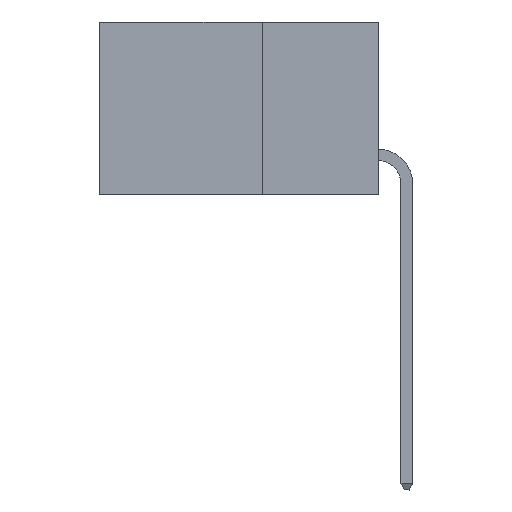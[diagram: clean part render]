
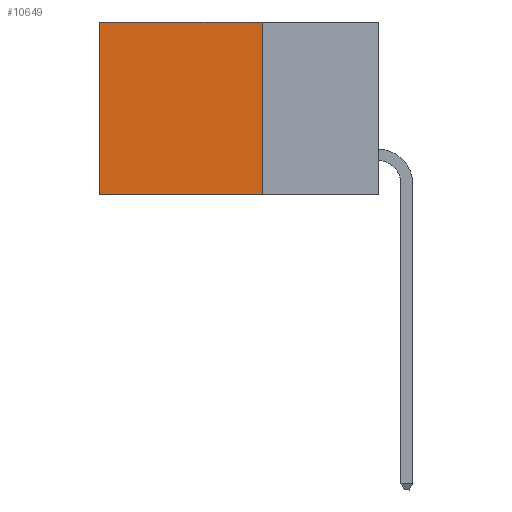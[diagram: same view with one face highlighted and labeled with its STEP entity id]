
A CAD part, left-side view. The second image highlights one B-rep face of the part: STEP entity #10649.
In plain terms, the highlighted planar face has unit normal (-1, 0, 0).
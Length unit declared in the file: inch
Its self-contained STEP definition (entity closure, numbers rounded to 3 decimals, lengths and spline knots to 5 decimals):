
#501 = ORIENTED_EDGE ( 'NONE', *, *, #8324, .F. ) ;
#2434 = VERTEX_POINT ( 'NONE', #20679 ) ;
#2759 = VERTEX_POINT ( 'NONE', #7507 ) ;
#4105 = PLANE ( 'NONE',  #6520 ) ;
#4493 = LINE ( 'NONE', #26517, #22009 ) ;
#4566 = EDGE_CURVE ( 'NONE', #2759, #28266, #4493, .T. ) ;
#5671 = EDGE_CURVE ( 'NONE', #2434, #25609, #22281, .T. ) ;
#6480 = DIRECTION ( 'NONE',  ( 0., 0., -1. ) ) ;
#6520 = AXIS2_PLACEMENT_3D ( 'NONE', #26674, #20231, #6480 ) ;
#7507 = CARTESIAN_POINT ( 'NONE',  ( 0.298, 0.6, 0. ) ) ;
#7579 = ORIENTED_EDGE ( 'NONE', *, *, #5671, .F. ) ;
#8324 = EDGE_CURVE ( 'NONE', #25609, #28266, #11415, .T. ) ;
#8355 = ORIENTED_EDGE ( 'NONE', *, *, #4566, .T. ) ;
#9033 = DIRECTION ( 'NONE',  ( 0., 0., -1. ) ) ;
#10649 = ADVANCED_FACE ( 'NONE', ( #23493 ), #4105, .F. ) ;
#11415 = LINE ( 'NONE', #25980, #16137 ) ;
#12291 = CARTESIAN_POINT ( 'NONE',  ( 0.298, 0.6, -0.37 ) ) ;
#13016 = CARTESIAN_POINT ( 'NONE',  ( 0.298, 0.25, 0. ) ) ;
#15783 = VECTOR ( 'NONE', #9033, 39.37008 ) ;
#16137 = VECTOR ( 'NONE', #28150, 39.37008 ) ;
#17869 = CARTESIAN_POINT ( 'NONE',  ( 0.298, 0.25, 0. ) ) ;
#18922 = EDGE_CURVE ( 'NONE', #2434, #2759, #28750, .T. ) ;
#18955 = ORIENTED_EDGE ( 'NONE', *, *, #18922, .T. ) ;
#20231 = DIRECTION ( 'NONE',  ( 1., 0., 0. ) ) ;
#20679 = CARTESIAN_POINT ( 'NONE',  ( 0.298, 0.25, 0. ) ) ;
#22009 = VECTOR ( 'NONE', #26482, 39.37008 ) ;
#22281 = LINE ( 'NONE', #13016, #15783 ) ;
#22938 = VECTOR ( 'NONE', #26604, 39.37008 ) ;
#23114 = EDGE_LOOP ( 'NONE', ( #8355, #501, #7579, #18955 ) ) ;
#23493 = FACE_OUTER_BOUND ( 'NONE', #23114, .T. ) ;
#25049 = CARTESIAN_POINT ( 'NONE',  ( 0.298, 0.25, -0.37 ) ) ;
#25609 = VERTEX_POINT ( 'NONE', #25049 ) ;
#25980 = CARTESIAN_POINT ( 'NONE',  ( 0.298, 0.25, -0.37 ) ) ;
#26482 = DIRECTION ( 'NONE',  ( 0., 0., -1. ) ) ;
#26517 = CARTESIAN_POINT ( 'NONE',  ( 0.298, 0.6, 0. ) ) ;
#26604 = DIRECTION ( 'NONE',  ( 0., 1., 0. ) ) ;
#26674 = CARTESIAN_POINT ( 'NONE',  ( 0.298, 0.25, 0. ) ) ;
#28150 = DIRECTION ( 'NONE',  ( 0., 1., 0. ) ) ;
#28266 = VERTEX_POINT ( 'NONE', #12291 ) ;
#28750 = LINE ( 'NONE', #17869, #22938 ) ;
